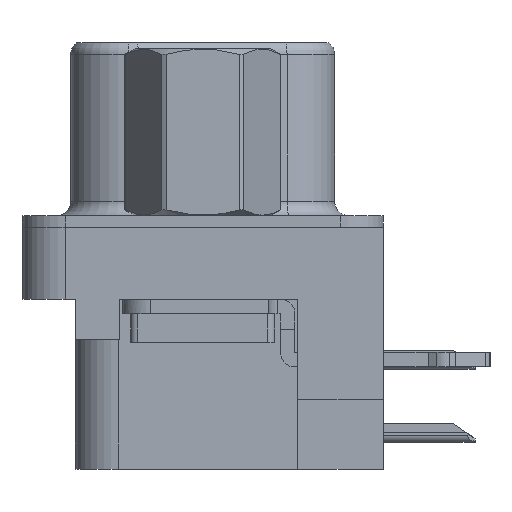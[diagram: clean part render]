
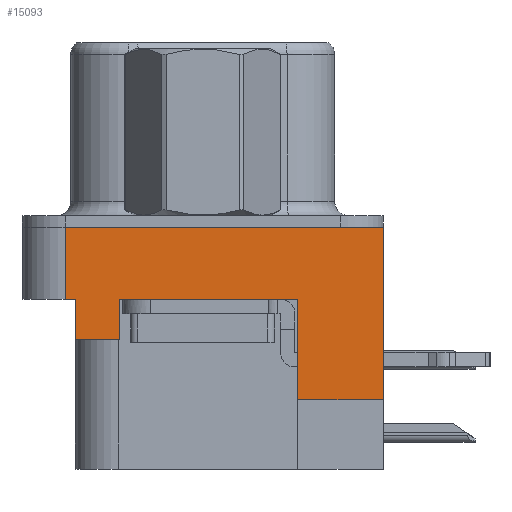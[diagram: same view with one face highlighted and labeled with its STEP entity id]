
A CAD part, left-side view. The second image highlights one B-rep face of the part: STEP entity #15093.
In plain terms, the highlighted planar face has unit normal (-1, 0, 0).
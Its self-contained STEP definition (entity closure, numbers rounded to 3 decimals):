
#726 = VERTEX_POINT ( 'NONE', #1229 ) ;
#814 = CARTESIAN_POINT ( 'NONE',  ( -3., 2.895, -2.5 ) ) ;
#984 = DIRECTION ( 'NONE',  ( 0., 0., 1. ) ) ;
#1114 = LINE ( 'NONE', #11348, #11790 ) ;
#1229 = CARTESIAN_POINT ( 'NONE',  ( -3., -3.295, -2.5 ) ) ;
#1454 = VECTOR ( 'NONE', #14890, 1000. ) ;
#1819 = VECTOR ( 'NONE', #22646, 1000. ) ;
#2410 = LINE ( 'NONE', #4822, #13167 ) ;
#2907 = DIRECTION ( 'NONE',  ( 0., 0., 1. ) ) ;
#3097 = DIRECTION ( 'NONE',  ( 0., 0., 1. ) ) ;
#3348 = CARTESIAN_POINT ( 'NONE',  ( -3., -6.275, -2.5 ) ) ;
#4706 = VECTOR ( 'NONE', #18071, 1000. ) ;
#4729 = LINE ( 'NONE', #12480, #14820 ) ;
#4822 = CARTESIAN_POINT ( 'NONE',  ( -3., -6.495, -6. ) ) ;
#4998 = DIRECTION ( 'NONE',  ( 0., -1., 0. ) ) ;
#5430 = ORIENTED_EDGE ( 'NONE', *, *, #21249, .F. ) ;
#5864 = VERTEX_POINT ( 'NONE', #17051 ) ;
#6696 = VERTEX_POINT ( 'NONE', #18102 ) ;
#6762 = CARTESIAN_POINT ( 'NONE',  ( -3., 4.425, -2.5 ) ) ;
#6906 = DIRECTION ( 'NONE',  ( 0., 1., 0. ) ) ;
#7339 = LINE ( 'NONE', #3348, #1819 ) ;
#7455 = PLANE ( 'NONE',  #10068 ) ;
#7691 = ORIENTED_EDGE ( 'NONE', *, *, #20974, .F. ) ;
#8425 = VERTEX_POINT ( 'NONE', #814 ) ;
#9638 = VERTEX_POINT ( 'NONE', #23932 ) ;
#9956 = VERTEX_POINT ( 'NONE', #12219 ) ;
#10068 = AXIS2_PLACEMENT_3D ( 'NONE', #24719, #11916, #26792 ) ;
#10333 = VERTEX_POINT ( 'NONE', #13796 ) ;
#11348 = CARTESIAN_POINT ( 'NONE',  ( -3., -6.275, 0. ) ) ;
#11394 = CARTESIAN_POINT ( 'NONE',  ( -3., 4.425, -3.9 ) ) ;
#11616 = EDGE_LOOP ( 'NONE', ( #5430, #26532, #27173, #22605, #15185, #14875, #7691, #23274, #18589, #21598 ) ) ;
#11790 = VECTOR ( 'NONE', #4998, 1000. ) ;
#11791 = DIRECTION ( 'NONE',  ( 0., 0., 1. ) ) ;
#11916 = DIRECTION ( 'NONE',  ( -1., 0., 0. ) ) ;
#12219 = CARTESIAN_POINT ( 'NONE',  ( -3., 2.895, -3.9 ) ) ;
#12472 = VECTOR ( 'NONE', #2907, 1000. ) ;
#12480 = CARTESIAN_POINT ( 'NONE',  ( -3., 4.425, -3.9 ) ) ;
#12774 = CARTESIAN_POINT ( 'NONE',  ( -3., -6.275, -2.5 ) ) ;
#13167 = VECTOR ( 'NONE', #6906, 1000. ) ;
#13796 = CARTESIAN_POINT ( 'NONE',  ( -3., -6.275, -6. ) ) ;
#14757 = VERTEX_POINT ( 'NONE', #6762 ) ;
#14794 = VECTOR ( 'NONE', #11791, 1000. ) ;
#14820 = VECTOR ( 'NONE', #18872, 1000. ) ;
#14875 = ORIENTED_EDGE ( 'NONE', *, *, #21358, .F. ) ;
#14890 = DIRECTION ( 'NONE',  ( 0., -1., 0. ) ) ;
#15093 = ADVANCED_FACE ( 'NONE', ( #22239 ), #7455, .T. ) ;
#15185 = ORIENTED_EDGE ( 'NONE', *, *, #21055, .T. ) ;
#15441 = LINE ( 'NONE', #20336, #14794 ) ;
#15696 = CARTESIAN_POINT ( 'NONE',  ( -3., -6.275, -2.5 ) ) ;
#15861 = CARTESIAN_POINT ( 'NONE',  ( -3., 4.425, -3.9 ) ) ;
#16093 = VECTOR ( 'NONE', #984, 1000. ) ;
#16846 = VECTOR ( 'NONE', #3097, 1000. ) ;
#16888 = VERTEX_POINT ( 'NONE', #26418 ) ;
#17051 = CARTESIAN_POINT ( 'NONE',  ( -3., -6.275, 0. ) ) ;
#17539 = LINE ( 'NONE', #18074, #16846 ) ;
#18071 = DIRECTION ( 'NONE',  ( 0., 0., 1. ) ) ;
#18074 = CARTESIAN_POINT ( 'NONE',  ( -3., 2.895, -3.9 ) ) ;
#18102 = CARTESIAN_POINT ( 'NONE',  ( -3., -3.295, -6. ) ) ;
#18589 = ORIENTED_EDGE ( 'NONE', *, *, #19749, .T. ) ;
#18872 = DIRECTION ( 'NONE',  ( 0., 1., 0. ) ) ;
#18988 = VERTEX_POINT ( 'NONE', #11394 ) ;
#19749 = EDGE_CURVE ( 'NONE', #8425, #726, #7339, .T. ) ;
#20336 = CARTESIAN_POINT ( 'NONE',  ( -3., -3.295, -8.4 ) ) ;
#20469 = EDGE_CURVE ( 'NONE', #9956, #8425, #17539, .T. ) ;
#20974 = EDGE_CURVE ( 'NONE', #9956, #18988, #4729, .T. ) ;
#21055 = EDGE_CURVE ( 'NONE', #16888, #14757, #25513, .T. ) ;
#21249 = EDGE_CURVE ( 'NONE', #10333, #6696, #2410, .T. ) ;
#21284 = EDGE_CURVE ( 'NONE', #10333, #5864, #23192, .T. ) ;
#21287 = EDGE_CURVE ( 'NONE', #9638, #5864, #1114, .T. ) ;
#21356 = EDGE_CURVE ( 'NONE', #16888, #9638, #27406, .T. ) ;
#21358 = EDGE_CURVE ( 'NONE', #18988, #14757, #21837, .T. ) ;
#21403 = EDGE_CURVE ( 'NONE', #6696, #726, #15441, .T. ) ;
#21598 = ORIENTED_EDGE ( 'NONE', *, *, #21403, .F. ) ;
#21837 = LINE ( 'NONE', #15861, #4706 ) ;
#22239 = FACE_OUTER_BOUND ( 'NONE', #11616, .T. ) ;
#22605 = ORIENTED_EDGE ( 'NONE', *, *, #21356, .F. ) ;
#22646 = DIRECTION ( 'NONE',  ( 0., -1., 0. ) ) ;
#23192 = LINE ( 'NONE', #15696, #12472 ) ;
#23274 = ORIENTED_EDGE ( 'NONE', *, *, #20469, .T. ) ;
#23932 = CARTESIAN_POINT ( 'NONE',  ( -3., 4.775, 0. ) ) ;
#24719 = CARTESIAN_POINT ( 'NONE',  ( -3., -6.275, -2.5 ) ) ;
#25513 = LINE ( 'NONE', #12774, #1454 ) ;
#26418 = CARTESIAN_POINT ( 'NONE',  ( -3., 4.775, -2.5 ) ) ;
#26490 = CARTESIAN_POINT ( 'NONE',  ( -3., 4.775, -2.5 ) ) ;
#26532 = ORIENTED_EDGE ( 'NONE', *, *, #21284, .T. ) ;
#26792 = DIRECTION ( 'NONE',  ( 0., 0., 1. ) ) ;
#27173 = ORIENTED_EDGE ( 'NONE', *, *, #21287, .F. ) ;
#27406 = LINE ( 'NONE', #26490, #16093 ) ;
